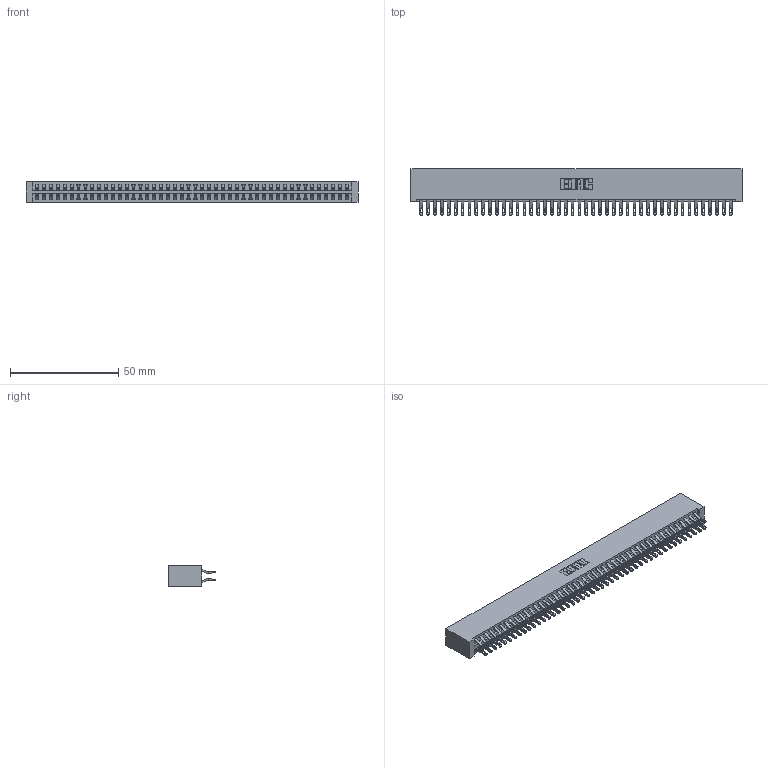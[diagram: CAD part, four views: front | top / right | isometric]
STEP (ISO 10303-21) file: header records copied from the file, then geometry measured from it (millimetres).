
FILE_DESCRIPTION (( 'STEP AP203' ), '1' );
FILE_NAME ('346-092-555-201.STEP', '2022-05-26T07:37:16', ( '' ), ( '' ), 'SwSTEP 2.0', 'SolidWorks 2020', '' );
FILE_SCHEMA (( 'CONFIG_CONTROL_DESIGN' ));
Length unit declared in the file: inch
Products named in the file (3): 345-292-001_555 Tail; 346 Part_No Mounting Lugs; 346-092-555-201
Assembly tree (93 placements, depth 2):
  346-092-555-201
    346 Part_No Mounting Lugs
    345-292-001_555 Tail  x92
Bounding box: 153.29 x 21.46 x 9.4 mm (x, y, z)
Volume: 15818.8 mm3; surface area: 22921.3 mm2
Topology: 93 solids, 93 shells, 5450 faces, 17141 edges, 11426 vertices
Faces by surface type: plane 3108, cylinder 2342
Entity records: 29531 total; most frequent: CARTESIAN_POINT 4894, ORIENTED_EDGE 4798, DIRECTION 4327, EDGE_CURVE 2399, LINE 2071, VECTOR 2071, VERTEX_POINT 1598, AXIS2_PLACEMENT_3D 1128
